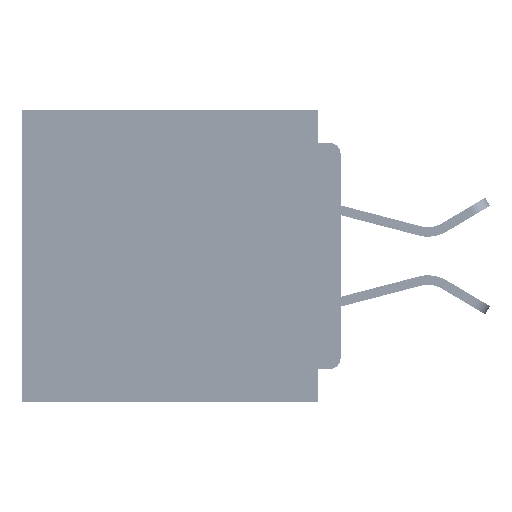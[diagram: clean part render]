
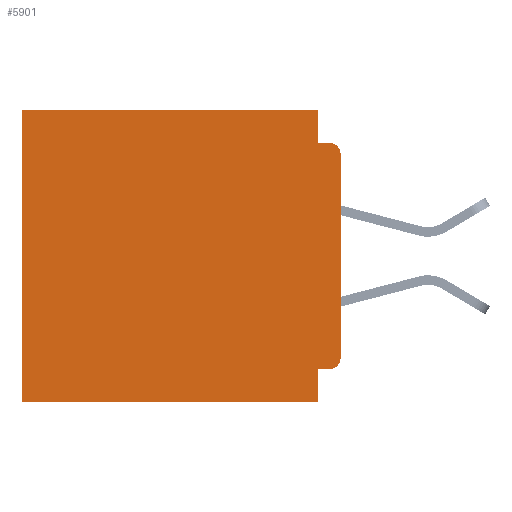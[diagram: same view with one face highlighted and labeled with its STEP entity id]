
A CAD part, left-side view. The second image highlights one B-rep face of the part: STEP entity #5901.
In plain terms, the highlighted planar face has unit normal (-1, 0, 0).
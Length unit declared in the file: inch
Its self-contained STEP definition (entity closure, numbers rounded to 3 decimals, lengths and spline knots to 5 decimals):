
#403 = VECTOR ( 'NONE', #17435, 39.37008 ) ;
#1306 = CARTESIAN_POINT ( 'NONE',  ( 0.3, 0., -0.34 ) ) ;
#1330 = LINE ( 'NONE', #48928, #30489 ) ;
#1964 = CARTESIAN_POINT ( 'NONE',  ( 0.3, 0., -0.4 ) ) ;
#2515 = CARTESIAN_POINT ( 'NONE',  ( 0.3, 0.015, -0.34 ) ) ;
#3924 = DIRECTION ( 'NONE',  ( 0., 0., -1. ) ) ;
#4083 = CARTESIAN_POINT ( 'NONE',  ( 0.3, 0.015, -0.045 ) ) ;
#4341 = ORIENTED_EDGE ( 'NONE', *, *, #15436, .F. ) ;
#4612 = AXIS2_PLACEMENT_3D ( 'NONE', #37138, #41078, #17443 ) ;
#5080 = VERTEX_POINT ( 'NONE', #27935 ) ;
#5473 = CARTESIAN_POINT ( 'NONE',  ( 0.3, 0., -0.355 ) ) ;
#5490 = VERTEX_POINT ( 'NONE', #42152 ) ;
#5788 = CIRCLE ( 'NONE', #35335, 0.015 ) ;
#5835 = VECTOR ( 'NONE', #3924, 39.37008 ) ;
#5901 = ADVANCED_FACE ( 'NONE', ( #29362 ), #9479, .F. ) ;
#5917 = ORIENTED_EDGE ( 'NONE', *, *, #49562, .T. ) ;
#6499 = DIRECTION ( 'NONE',  ( 0., 0., -1. ) ) ;
#6563 = VECTOR ( 'NONE', #45550, 39.37008 ) ;
#6801 = LINE ( 'NONE', #1964, #26664 ) ;
#7805 = LINE ( 'NONE', #33979, #6563 ) ;
#9295 = CARTESIAN_POINT ( 'NONE',  ( 0.3, 0., 0. ) ) ;
#9479 = PLANE ( 'NONE',  #4612 ) ;
#10560 = DIRECTION ( 'NONE',  ( -1., 0., 0. ) ) ;
#11368 = VERTEX_POINT ( 'NONE', #1306 ) ;
#12234 = LINE ( 'NONE', #9295, #403 ) ;
#12879 = ORIENTED_EDGE ( 'NONE', *, *, #43500, .F. ) ;
#13948 = CARTESIAN_POINT ( 'NONE',  ( 0.3, 0., -0.06 ) ) ;
#14968 = CARTESIAN_POINT ( 'NONE',  ( 0.3, 0.031, -0.355 ) ) ;
#15077 = VERTEX_POINT ( 'NONE', #26327 ) ;
#15144 = LINE ( 'NONE', #27711, #5835 ) ;
#15436 = EDGE_CURVE ( 'NONE', #29021, #40715, #29260, .T. ) ;
#16820 = VECTOR ( 'NONE', #46668, 39.37008 ) ;
#16936 = EDGE_CURVE ( 'NONE', #24210, #22038, #32210, .T. ) ;
#17435 = DIRECTION ( 'NONE',  ( 0., 1., 0. ) ) ;
#17443 = DIRECTION ( 'NONE',  ( 0., 0., -1. ) ) ;
#17920 = DIRECTION ( 'NONE',  ( 0., 0., -1. ) ) ;
#18074 = LINE ( 'NONE', #42812, #16820 ) ;
#20570 = CARTESIAN_POINT ( 'NONE',  ( 0.3, 0.031, -0.045 ) ) ;
#21162 = DIRECTION ( 'NONE',  ( 0., 0., -1. ) ) ;
#22038 = VERTEX_POINT ( 'NONE', #4083 ) ;
#22226 = ORIENTED_EDGE ( 'NONE', *, *, #32703, .T. ) ;
#23518 = ORIENTED_EDGE ( 'NONE', *, *, #41183, .F. ) ;
#24210 = VERTEX_POINT ( 'NONE', #13948 ) ;
#24300 = CARTESIAN_POINT ( 'NONE',  ( 0.3, 0.015, -0.355 ) ) ;
#26327 = CARTESIAN_POINT ( 'NONE',  ( 0.3, 0.437, -0.4 ) ) ;
#26664 = VECTOR ( 'NONE', #17920, 39.37008 ) ;
#27711 = CARTESIAN_POINT ( 'NONE',  ( 0.3, 0.031, -0.4 ) ) ;
#27935 = CARTESIAN_POINT ( 'NONE',  ( 0.3, 0.031, 0. ) ) ;
#28573 = VECTOR ( 'NONE', #21162, 39.37008 ) ;
#28658 = EDGE_LOOP ( 'NONE', ( #38069, #46992, #23518, #29376, #22226, #33263, #12879, #46719, #4341, #5917 ) ) ;
#28943 = CARTESIAN_POINT ( 'NONE',  ( 0.3, 0.031, 0. ) ) ;
#29021 = VERTEX_POINT ( 'NONE', #24300 ) ;
#29260 = LINE ( 'NONE', #5473, #38499 ) ;
#29362 = FACE_OUTER_BOUND ( 'NONE', #28658, .T. ) ;
#29376 = ORIENTED_EDGE ( 'NONE', *, *, #51028, .F. ) ;
#29504 = DIRECTION ( 'NONE',  ( 0., 1., 0. ) ) ;
#30251 = DIRECTION ( 'NONE',  ( -1., 0., 0. ) ) ;
#30489 = VECTOR ( 'NONE', #29504, 39.37008 ) ;
#30503 = EDGE_CURVE ( 'NONE', #24210, #11368, #6801, .T. ) ;
#30708 = VERTEX_POINT ( 'NONE', #20570 ) ;
#32210 = CIRCLE ( 'NONE', #38442, 0.015 ) ;
#32703 = EDGE_CURVE ( 'NONE', #5080, #5490, #12234, .T. ) ;
#33263 = ORIENTED_EDGE ( 'NONE', *, *, #44462, .T. ) ;
#33979 = CARTESIAN_POINT ( 'NONE',  ( 0.3, 0., -0.045 ) ) ;
#34268 = CARTESIAN_POINT ( 'NONE',  ( 0.3, 0.015, -0.06 ) ) ;
#35335 = AXIS2_PLACEMENT_3D ( 'NONE', #2515, #30251, #6499 ) ;
#37138 = CARTESIAN_POINT ( 'NONE',  ( 0.3, 0., -0.4 ) ) ;
#38069 = ORIENTED_EDGE ( 'NONE', *, *, #30503, .F. ) ;
#38180 = DIRECTION ( 'NONE',  ( 0., 0., -1. ) ) ;
#38442 = AXIS2_PLACEMENT_3D ( 'NONE', #34268, #10560, #38180 ) ;
#38499 = VECTOR ( 'NONE', #40912, 39.37008 ) ;
#39042 = LINE ( 'NONE', #28943, #28573 ) ;
#40715 = VERTEX_POINT ( 'NONE', #14968 ) ;
#40912 = DIRECTION ( 'NONE',  ( 0., 1., 0. ) ) ;
#41078 = DIRECTION ( 'NONE',  ( 1., 0., 0. ) ) ;
#41183 = EDGE_CURVE ( 'NONE', #30708, #22038, #7805, .T. ) ;
#42152 = CARTESIAN_POINT ( 'NONE',  ( 0.3, 0.437, 0. ) ) ;
#42812 = CARTESIAN_POINT ( 'NONE',  ( 0.3, 0.437, -0.4 ) ) ;
#43500 = EDGE_CURVE ( 'NONE', #49743, #15077, #1330, .T. ) ;
#44462 = EDGE_CURVE ( 'NONE', #5490, #15077, #18074, .T. ) ;
#45550 = DIRECTION ( 'NONE',  ( 0., -1., 0. ) ) ;
#46668 = DIRECTION ( 'NONE',  ( 0., 0., -1. ) ) ;
#46719 = ORIENTED_EDGE ( 'NONE', *, *, #49155, .F. ) ;
#46992 = ORIENTED_EDGE ( 'NONE', *, *, #16936, .T. ) ;
#48928 = CARTESIAN_POINT ( 'NONE',  ( 0.3, 0., -0.4 ) ) ;
#49155 = EDGE_CURVE ( 'NONE', #40715, #49743, #15144, .T. ) ;
#49562 = EDGE_CURVE ( 'NONE', #29021, #11368, #5788, .T. ) ;
#49743 = VERTEX_POINT ( 'NONE', #50814 ) ;
#50814 = CARTESIAN_POINT ( 'NONE',  ( 0.3, 0.031, -0.4 ) ) ;
#51028 = EDGE_CURVE ( 'NONE', #5080, #30708, #39042, .T. ) ;
